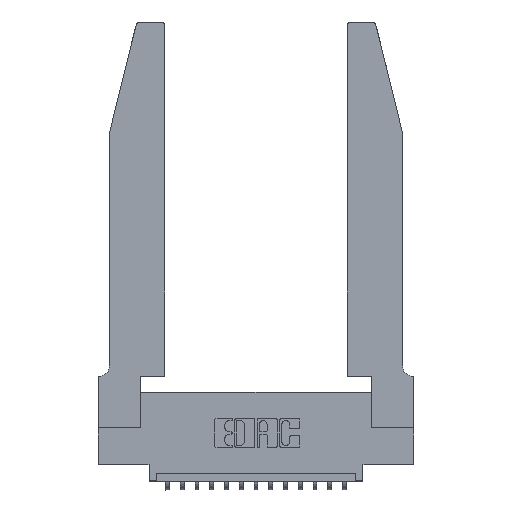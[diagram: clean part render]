
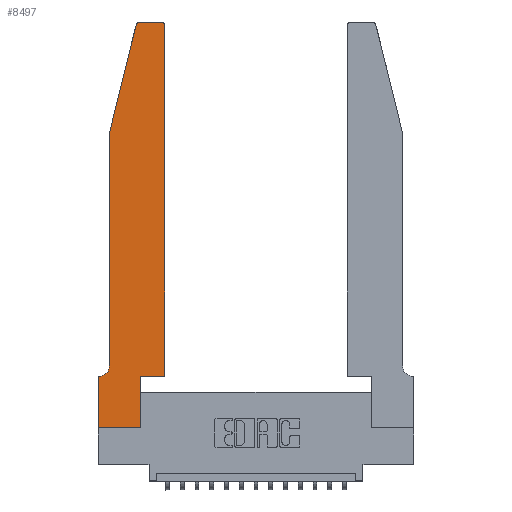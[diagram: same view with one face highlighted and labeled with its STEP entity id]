
A CAD part, top view. The second image highlights one B-rep face of the part: STEP entity #8497.
In plain terms, the highlighted planar face has unit normal (0, 0, 1).
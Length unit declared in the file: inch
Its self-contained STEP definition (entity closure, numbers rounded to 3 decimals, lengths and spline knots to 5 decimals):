
#374 = AXIS2_PLACEMENT_3D ( 'NONE', #992, #2447, #2885 ) ;
#445 = ORIENTED_EDGE ( 'NONE', *, *, #2448, .T. ) ;
#524 = CARTESIAN_POINT ( 'NONE',  ( 0.4505, 0.35, 0.37 ) ) ;
#891 = EDGE_CURVE ( 'NONE', #9117, #8923, #4481, .T. ) ;
#921 = EDGE_CURVE ( 'NONE', #11125, #1254, #12989, .T. ) ;
#944 = EDGE_CURVE ( 'NONE', #3469, #9117, #6722, .T. ) ;
#992 = CARTESIAN_POINT ( 'NONE',  ( 0.4205, 2.72, 0.37 ) ) ;
#1058 = CARTESIAN_POINT ( 'NONE',  ( 0., 0., 0.37 ) ) ;
#1087 = CARTESIAN_POINT ( 'NONE',  ( 0.4205, 2.75, 0.37 ) ) ;
#1254 = VERTEX_POINT ( 'NONE', #18297 ) ;
#1863 = CIRCLE ( 'NONE', #15068, 0.07 ) ;
#2264 = ORIENTED_EDGE ( 'NONE', *, *, #17434, .T. ) ;
#2341 = CARTESIAN_POINT ( 'NONE',  ( 0.4505, 0.35, 0.37 ) ) ;
#2447 = DIRECTION ( 'NONE',  ( 0., 0., 1. ) ) ;
#2448 = EDGE_CURVE ( 'NONE', #1254, #12007, #7658, .T. ) ;
#2678 = EDGE_CURVE ( 'NONE', #16498, #3469, #5188, .T. ) ;
#2719 = EDGE_CURVE ( 'NONE', #2879, #11125, #13677, .T. ) ;
#2777 = DIRECTION ( 'NONE',  ( 0., -1., 0. ) ) ;
#2879 = VERTEX_POINT ( 'NONE', #1087 ) ;
#2885 = DIRECTION ( 'NONE',  ( 1., 0., 0. ) ) ;
#2977 = ORIENTED_EDGE ( 'NONE', *, *, #12750, .T. ) ;
#3210 = ORIENTED_EDGE ( 'NONE', *, *, #7371, .T. ) ;
#3246 = LINE ( 'NONE', #524, #6606 ) ;
#3469 = VERTEX_POINT ( 'NONE', #15256 ) ;
#3736 = LINE ( 'NONE', #2341, #9343 ) ;
#3766 = DIRECTION ( 'NONE',  ( 0., -1., 0. ) ) ;
#4079 = EDGE_CURVE ( 'NONE', #11724, #2879, #12325, .T. ) ;
#4111 = VERTEX_POINT ( 'NONE', #18153 ) ;
#4469 = VERTEX_POINT ( 'NONE', #8138 ) ;
#4481 = LINE ( 'NONE', #12142, #15426 ) ;
#4541 = DIRECTION ( 'NONE',  ( 0., 0., 1. ) ) ;
#4894 = CARTESIAN_POINT ( 'NONE',  ( 0.284, 2.75, 0.37 ) ) ;
#5188 = LINE ( 'NONE', #10357, #5645 ) ;
#5374 = VECTOR ( 'NONE', #2777, 39.37008 ) ;
#5645 = VECTOR ( 'NONE', #7462, 39.37008 ) ;
#5878 = CARTESIAN_POINT ( 'NONE',  ( 0.0755, 2., 0.37 ) ) ;
#5941 = CARTESIAN_POINT ( 'NONE',  ( 0.0055, 0.35, 0.37 ) ) ;
#5978 = EDGE_CURVE ( 'NONE', #4469, #14610, #3736, .T. ) ;
#6068 = CARTESIAN_POINT ( 'NONE',  ( 0.2865, 0.35, 0.37 ) ) ;
#6544 = AXIS2_PLACEMENT_3D ( 'NONE', #6603, #6662, #16608 ) ;
#6599 = VECTOR ( 'NONE', #17422, 39.37008 ) ;
#6603 = CARTESIAN_POINT ( 'NONE',  ( 0.284, 2.72, 0.37 ) ) ;
#6606 = VECTOR ( 'NONE', #10552, 39.37008 ) ;
#6662 = DIRECTION ( 'NONE',  ( 0., 0., 1. ) ) ;
#6722 = LINE ( 'NONE', #1058, #5374 ) ;
#6741 = ORIENTED_EDGE ( 'NONE', *, *, #891, .T. ) ;
#7261 = PLANE ( 'NONE',  #14963 ) ;
#7281 = EDGE_CURVE ( 'NONE', #8923, #4469, #16438, .T. ) ;
#7371 = EDGE_CURVE ( 'NONE', #4111, #16498, #1863, .T. ) ;
#7462 = DIRECTION ( 'NONE',  ( -1., 0., 0. ) ) ;
#7658 = LINE ( 'NONE', #17060, #14797 ) ;
#8138 = CARTESIAN_POINT ( 'NONE',  ( 0.2865, 0.35, 0.37 ) ) ;
#8497 = ADVANCED_FACE ( 'NONE', ( #17996 ), #7261, .T. ) ;
#8796 = CARTESIAN_POINT ( 'NONE',  ( 0., 0.35, 0.37 ) ) ;
#8923 = VERTEX_POINT ( 'NONE', #17965 ) ;
#9057 = ORIENTED_EDGE ( 'NONE', *, *, #7281, .T. ) ;
#9117 = VERTEX_POINT ( 'NONE', #14709 ) ;
#9155 = ORIENTED_EDGE ( 'NONE', *, *, #2678, .T. ) ;
#9343 = VECTOR ( 'NONE', #13652, 39.37008 ) ;
#9709 = DIRECTION ( 'NONE',  ( -0.239, -0.971, 0. ) ) ;
#9892 = VECTOR ( 'NONE', #12328, 39.37008 ) ;
#10357 = CARTESIAN_POINT ( 'NONE',  ( 0.0755, 0.35, 0.37 ) ) ;
#10461 = DIRECTION ( 'NONE',  ( 1., 0., 0. ) ) ;
#10552 = DIRECTION ( 'NONE',  ( 0., 1., 0. ) ) ;
#11125 = VERTEX_POINT ( 'NONE', #4894 ) ;
#11199 = CARTESIAN_POINT ( 'NONE',  ( 0.0055, 0.42, 0.37 ) ) ;
#11724 = VERTEX_POINT ( 'NONE', #13247 ) ;
#12007 = VERTEX_POINT ( 'NONE', #5878 ) ;
#12142 = CARTESIAN_POINT ( 'NONE',  ( 0., 0., 0.37 ) ) ;
#12325 = CIRCLE ( 'NONE', #374, 0.03 ) ;
#12328 = DIRECTION ( 'NONE',  ( -1., 0., 0. ) ) ;
#12588 = DIRECTION ( 'NONE',  ( 0., 0., -1. ) ) ;
#12750 = EDGE_CURVE ( 'NONE', #14610, #11724, #3246, .T. ) ;
#12989 = CIRCLE ( 'NONE', #6544, 0.03 ) ;
#13168 = DIRECTION ( 'NONE',  ( 1., 0., 0. ) ) ;
#13247 = CARTESIAN_POINT ( 'NONE',  ( 0.4505, 2.72, 0.37 ) ) ;
#13652 = DIRECTION ( 'NONE',  ( 1., 0., 0. ) ) ;
#13676 = CARTESIAN_POINT ( 'NONE',  ( 0.2605, 2.75, 0.37 ) ) ;
#13677 = LINE ( 'NONE', #13676, #9892 ) ;
#13737 = ORIENTED_EDGE ( 'NONE', *, *, #4079, .T. ) ;
#14008 = DIRECTION ( 'NONE',  ( -1., 0., 0. ) ) ;
#14306 = EDGE_LOOP ( 'NONE', ( #17357, #17389, #445, #2264, #3210, #9155, #15754, #6741, #9057, #17239, #2977, #13737 ) ) ;
#14610 = VERTEX_POINT ( 'NONE', #15513 ) ;
#14709 = CARTESIAN_POINT ( 'NONE',  ( 0., 0., 0.37 ) ) ;
#14797 = VECTOR ( 'NONE', #9709, 39.37008 ) ;
#14935 = LINE ( 'NONE', #15135, #18595 ) ;
#14963 = AXIS2_PLACEMENT_3D ( 'NONE', #8796, #4541, #13168 ) ;
#15068 = AXIS2_PLACEMENT_3D ( 'NONE', #11199, #12588, #14008 ) ;
#15135 = CARTESIAN_POINT ( 'NONE',  ( 0.0755, 2., 0.37 ) ) ;
#15256 = CARTESIAN_POINT ( 'NONE',  ( 0., 0.35, 0.37 ) ) ;
#15426 = VECTOR ( 'NONE', #10461, 39.37008 ) ;
#15513 = CARTESIAN_POINT ( 'NONE',  ( 0.4505, 0.35, 0.37 ) ) ;
#15754 = ORIENTED_EDGE ( 'NONE', *, *, #944, .T. ) ;
#16438 = LINE ( 'NONE', #6068, #6599 ) ;
#16498 = VERTEX_POINT ( 'NONE', #5941 ) ;
#16608 = DIRECTION ( 'NONE',  ( 1., 0., 0. ) ) ;
#17060 = CARTESIAN_POINT ( 'NONE',  ( 0.0755, 2., 0.37 ) ) ;
#17239 = ORIENTED_EDGE ( 'NONE', *, *, #5978, .T. ) ;
#17357 = ORIENTED_EDGE ( 'NONE', *, *, #2719, .T. ) ;
#17389 = ORIENTED_EDGE ( 'NONE', *, *, #921, .T. ) ;
#17422 = DIRECTION ( 'NONE',  ( 0., 1., 0. ) ) ;
#17434 = EDGE_CURVE ( 'NONE', #12007, #4111, #14935, .T. ) ;
#17965 = CARTESIAN_POINT ( 'NONE',  ( 0.2865, 0., 0.37 ) ) ;
#17996 = FACE_OUTER_BOUND ( 'NONE', #14306, .T. ) ;
#18153 = CARTESIAN_POINT ( 'NONE',  ( 0.0755, 0.42, 0.37 ) ) ;
#18297 = CARTESIAN_POINT ( 'NONE',  ( 0.25487, 2.72718, 0.37 ) ) ;
#18595 = VECTOR ( 'NONE', #3766, 39.37008 ) ;
